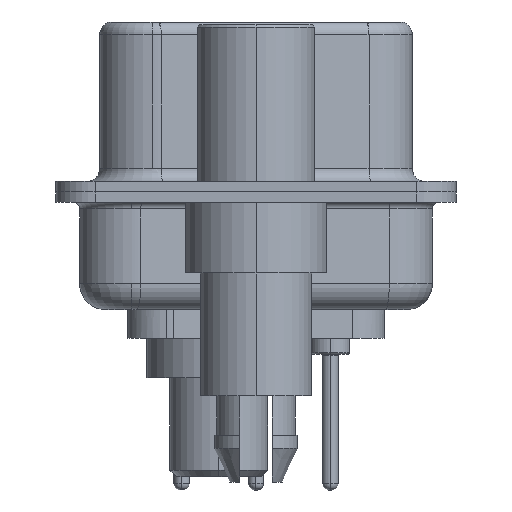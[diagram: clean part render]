
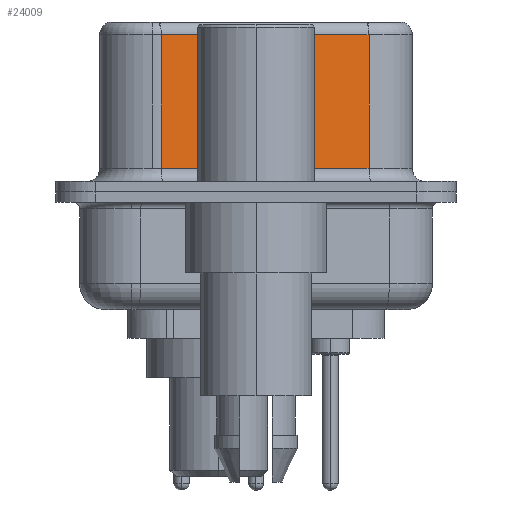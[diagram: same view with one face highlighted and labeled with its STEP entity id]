
A CAD part, left-side view. The second image highlights one B-rep face of the part: STEP entity #24009.
In plain terms, the highlighted planar face has unit normal (-0.985, -0.174, 0).
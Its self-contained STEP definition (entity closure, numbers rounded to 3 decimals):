
#42 = AXIS2_PLACEMENT_3D ( 'NONE', #5207, #28223, #14478 ) ;
#1504 = CARTESIAN_POINT ( 'NONE',  ( 3.73, 3.628, 6.02 ) ) ;
#1841 = CARTESIAN_POINT ( 'NONE',  ( 5.132, -4.322, 6.52 ) ) ;
#1944 = DIRECTION ( 'NONE',  ( 0., 0., -1. ) ) ;
#2740 = LINE ( 'NONE', #1841, #26527 ) ;
#3237 = ORIENTED_EDGE ( 'NONE', *, *, #7783, .T. ) ;
#5207 = CARTESIAN_POINT ( 'NONE',  ( 5.132, -4.322, 6.52 ) ) ;
#5911 = VERTEX_POINT ( 'NONE', #1504 ) ;
#6677 = CARTESIAN_POINT ( 'NONE',  ( 5.132, -4.322, 6.02 ) ) ;
#7588 = VECTOR ( 'NONE', #22907, 1000. ) ;
#7783 = EDGE_CURVE ( 'NONE', #25449, #5911, #20765, .T. ) ;
#7885 = VERTEX_POINT ( 'NONE', #9326 ) ;
#9326 = CARTESIAN_POINT ( 'NONE',  ( 3.73, 3.628, 0.9 ) ) ;
#10071 = CARTESIAN_POINT ( 'NONE',  ( 5.132, -4.322, 0.9 ) ) ;
#10646 = ORIENTED_EDGE ( 'NONE', *, *, #20086, .T. ) ;
#12202 = PLANE ( 'NONE',  #42 ) ;
#12766 = VERTEX_POINT ( 'NONE', #10071 ) ;
#14478 = DIRECTION ( 'NONE',  ( -0.174, 0.985, 0. ) ) ;
#15592 = CARTESIAN_POINT ( 'NONE',  ( 5.132, -4.322, 6.02 ) ) ;
#15974 = CARTESIAN_POINT ( 'NONE',  ( 5.132, -4.322, 0.9 ) ) ;
#17763 = VECTOR ( 'NONE', #22747, 1000. ) ;
#18065 = CARTESIAN_POINT ( 'NONE',  ( 3.73, 3.628, 6.52 ) ) ;
#18284 = VECTOR ( 'NONE', #29596, 1000. ) ;
#18367 = LINE ( 'NONE', #15974, #7588 ) ;
#18673 = EDGE_CURVE ( 'NONE', #7885, #12766, #18367, .T. ) ;
#20086 = EDGE_CURVE ( 'NONE', #5911, #7885, #24350, .T. ) ;
#20765 = LINE ( 'NONE', #6677, #17763 ) ;
#21752 = EDGE_CURVE ( 'NONE', #25449, #12766, #2740, .T. ) ;
#22747 = DIRECTION ( 'NONE',  ( -0.174, 0.985, 0. ) ) ;
#22907 = DIRECTION ( 'NONE',  ( 0.174, -0.985, 0. ) ) ;
#22939 = ORIENTED_EDGE ( 'NONE', *, *, #21752, .F. ) ;
#24009 = ADVANCED_FACE ( 'NONE', ( #27143 ), #12202, .F. ) ;
#24047 = EDGE_LOOP ( 'NONE', ( #22939, #3237, #10646, #25563 ) ) ;
#24350 = LINE ( 'NONE', #18065, #18284 ) ;
#25449 = VERTEX_POINT ( 'NONE', #15592 ) ;
#25563 = ORIENTED_EDGE ( 'NONE', *, *, #18673, .T. ) ;
#26527 = VECTOR ( 'NONE', #1944, 1000. ) ;
#27143 = FACE_OUTER_BOUND ( 'NONE', #24047, .T. ) ;
#28223 = DIRECTION ( 'NONE',  ( 0.985, 0.174, 0. ) ) ;
#29596 = DIRECTION ( 'NONE',  ( 0., 0., -1. ) ) ;
